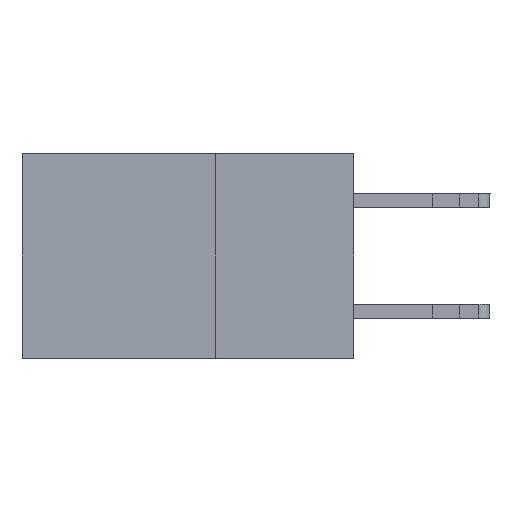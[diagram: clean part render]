
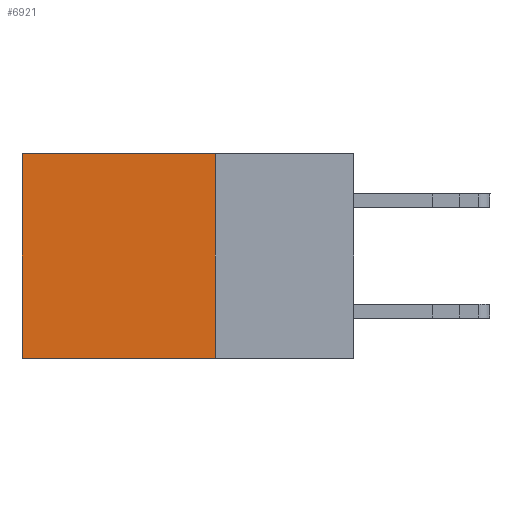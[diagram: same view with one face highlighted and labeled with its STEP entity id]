
A CAD part, left-side view. The second image highlights one B-rep face of the part: STEP entity #6921.
In plain terms, the highlighted planar face has unit normal (-1, 0, 0).
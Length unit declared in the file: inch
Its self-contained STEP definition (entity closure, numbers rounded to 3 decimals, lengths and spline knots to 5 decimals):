
#9 = CARTESIAN_POINT ( 'NONE',  ( 0.2875, 0.25, -0.37 ) ) ;
#435 = DIRECTION ( 'NONE',  ( 1., 0., 0. ) ) ;
#546 = EDGE_CURVE ( 'NONE', #19056, #19602, #18554, .T. ) ;
#635 = LINE ( 'NONE', #8084, #4507 ) ;
#2354 = VERTEX_POINT ( 'NONE', #4038 ) ;
#2806 = FACE_OUTER_BOUND ( 'NONE', #17776, .T. ) ;
#2887 = ORIENTED_EDGE ( 'NONE', *, *, #10735, .T. ) ;
#3006 = ORIENTED_EDGE ( 'NONE', *, *, #23318, .F. ) ;
#4038 = CARTESIAN_POINT ( 'NONE',  ( 0.2875, 0.25, 0. ) ) ;
#4222 = DIRECTION ( 'NONE',  ( 0., 1., 0. ) ) ;
#4507 = VECTOR ( 'NONE', #13786, 39.37008 ) ;
#5626 = CARTESIAN_POINT ( 'NONE',  ( 0.2875, 0.6, 0. ) ) ;
#5682 = CARTESIAN_POINT ( 'NONE',  ( 0.2875, 0.6, -0.37 ) ) ;
#6921 = ADVANCED_FACE ( 'NONE', ( #2806 ), #11808, .F. ) ;
#7120 = CARTESIAN_POINT ( 'NONE',  ( 0.2875, 0.25, 0. ) ) ;
#7868 = CARTESIAN_POINT ( 'NONE',  ( 0.2875, 0.25, -0.37 ) ) ;
#8022 = CARTESIAN_POINT ( 'NONE',  ( 0.2875, 0.25, 0. ) ) ;
#8084 = CARTESIAN_POINT ( 'NONE',  ( 0.2875, 0.25, 0. ) ) ;
#9012 = DIRECTION ( 'NONE',  ( 0., 0., -1. ) ) ;
#9252 = LINE ( 'NONE', #24357, #24247 ) ;
#10490 = EDGE_CURVE ( 'NONE', #23471, #19602, #9252, .T. ) ;
#10735 = EDGE_CURVE ( 'NONE', #2354, #23471, #635, .T. ) ;
#11808 = PLANE ( 'NONE',  #23824 ) ;
#12946 = VECTOR ( 'NONE', #4222, 39.37008 ) ;
#13114 = DIRECTION ( 'NONE',  ( 0., 0., -1. ) ) ;
#13719 = DIRECTION ( 'NONE',  ( 0., 0., -1. ) ) ;
#13786 = DIRECTION ( 'NONE',  ( 0., 1., 0. ) ) ;
#13890 = ORIENTED_EDGE ( 'NONE', *, *, #546, .F. ) ;
#14523 = LINE ( 'NONE', #7120, #23901 ) ;
#17776 = EDGE_LOOP ( 'NONE', ( #21682, #13890, #3006, #2887 ) ) ;
#18554 = LINE ( 'NONE', #7868, #12946 ) ;
#19056 = VERTEX_POINT ( 'NONE', #9 ) ;
#19602 = VERTEX_POINT ( 'NONE', #5682 ) ;
#21682 = ORIENTED_EDGE ( 'NONE', *, *, #10490, .T. ) ;
#23318 = EDGE_CURVE ( 'NONE', #2354, #19056, #14523, .T. ) ;
#23471 = VERTEX_POINT ( 'NONE', #5626 ) ;
#23824 = AXIS2_PLACEMENT_3D ( 'NONE', #8022, #435, #13719 ) ;
#23901 = VECTOR ( 'NONE', #9012, 39.37008 ) ;
#24247 = VECTOR ( 'NONE', #13114, 39.37008 ) ;
#24357 = CARTESIAN_POINT ( 'NONE',  ( 0.2875, 0.6, 0. ) ) ;
